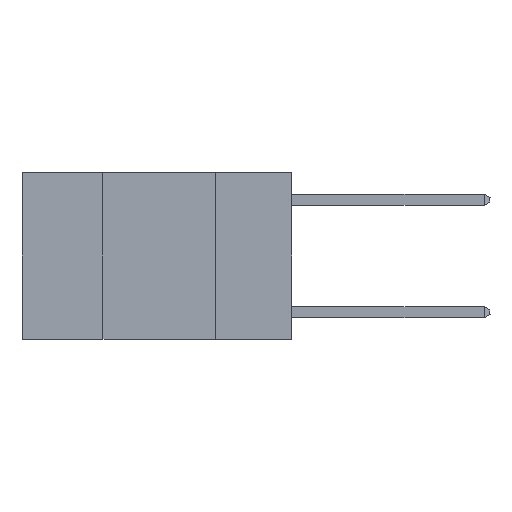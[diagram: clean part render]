
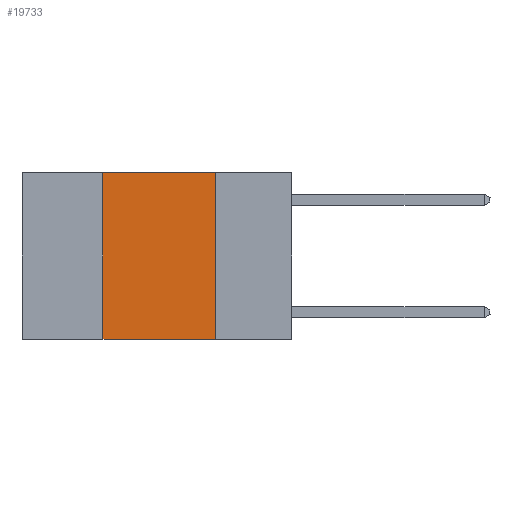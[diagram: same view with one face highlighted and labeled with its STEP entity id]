
A CAD part, left-side view. The second image highlights one B-rep face of the part: STEP entity #19733.
In plain terms, the highlighted planar face has unit normal (-1, 0, 0).
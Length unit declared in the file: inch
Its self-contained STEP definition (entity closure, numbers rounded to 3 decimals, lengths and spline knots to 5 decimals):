
#795 = CARTESIAN_POINT ( 'NONE',  ( 0., 0.6, 0. ) ) ;
#1106 = LINE ( 'NONE', #3116, #1187 ) ;
#1187 = VECTOR ( 'NONE', #11206, 39.37008 ) ;
#3116 = CARTESIAN_POINT ( 'NONE',  ( 0., 0.42, 0. ) ) ;
#3566 = ORIENTED_EDGE ( 'NONE', *, *, #25223, .F. ) ;
#4639 = VERTEX_POINT ( 'NONE', #25200 ) ;
#4696 = EDGE_CURVE ( 'NONE', #12910, #12222, #25447, .T. ) ;
#4785 = FACE_OUTER_BOUND ( 'NONE', #18239, .T. ) ;
#7161 = CARTESIAN_POINT ( 'NONE',  ( 0., 0.6, 0. ) ) ;
#7251 = VECTOR ( 'NONE', #14200, 39.37008 ) ;
#7283 = CARTESIAN_POINT ( 'NONE',  ( 0., 0.17, 0. ) ) ;
#7301 = DIRECTION ( 'NONE',  ( 0., -1., 0. ) ) ;
#9030 = DIRECTION ( 'NONE',  ( 0., 0., -1. ) ) ;
#11206 = DIRECTION ( 'NONE',  ( 0., 0., 1. ) ) ;
#12186 = LINE ( 'NONE', #24277, #7251 ) ;
#12222 = VERTEX_POINT ( 'NONE', #15542 ) ;
#12594 = CARTESIAN_POINT ( 'NONE',  ( 0., 0.42, 0. ) ) ;
#12736 = DIRECTION ( 'NONE',  ( 0., 0., -1. ) ) ;
#12910 = VERTEX_POINT ( 'NONE', #12594 ) ;
#13643 = LINE ( 'NONE', #7283, #16133 ) ;
#14200 = DIRECTION ( 'NONE',  ( 0., -1., 0. ) ) ;
#15007 = DIRECTION ( 'NONE',  ( 1., 0., 0. ) ) ;
#15356 = VERTEX_POINT ( 'NONE', #22431 ) ;
#15542 = CARTESIAN_POINT ( 'NONE',  ( 0., 0.17, 0. ) ) ;
#15599 = ORIENTED_EDGE ( 'NONE', *, *, #23175, .F. ) ;
#15925 = VECTOR ( 'NONE', #7301, 39.37008 ) ;
#16133 = VECTOR ( 'NONE', #9030, 39.37008 ) ;
#17822 = ORIENTED_EDGE ( 'NONE', *, *, #26114, .T. ) ;
#18149 = ORIENTED_EDGE ( 'NONE', *, *, #4696, .F. ) ;
#18239 = EDGE_LOOP ( 'NONE', ( #3566, #18149, #15599, #17822 ) ) ;
#19733 = ADVANCED_FACE ( 'NONE', ( #4785 ), #22585, .F. ) ;
#21905 = AXIS2_PLACEMENT_3D ( 'NONE', #795, #15007, #12736 ) ;
#22431 = CARTESIAN_POINT ( 'NONE',  ( 0., 0.17, -0.37 ) ) ;
#22585 = PLANE ( 'NONE',  #21905 ) ;
#23175 = EDGE_CURVE ( 'NONE', #4639, #12910, #1106, .T. ) ;
#24277 = CARTESIAN_POINT ( 'NONE',  ( 0., 0.6, -0.37 ) ) ;
#25200 = CARTESIAN_POINT ( 'NONE',  ( 0., 0.42, -0.37 ) ) ;
#25223 = EDGE_CURVE ( 'NONE', #12222, #15356, #13643, .T. ) ;
#25447 = LINE ( 'NONE', #7161, #15925 ) ;
#26114 = EDGE_CURVE ( 'NONE', #4639, #15356, #12186, .T. ) ;
